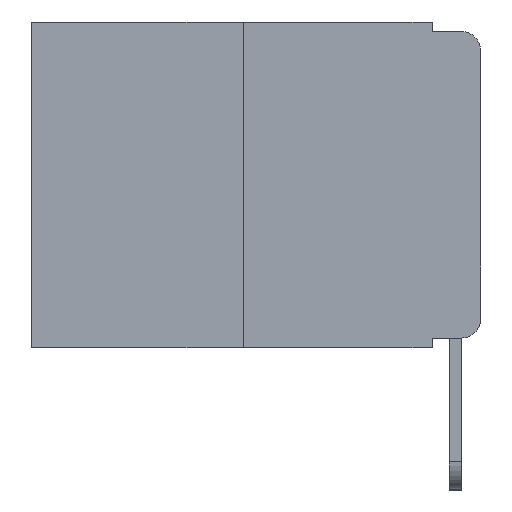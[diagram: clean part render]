
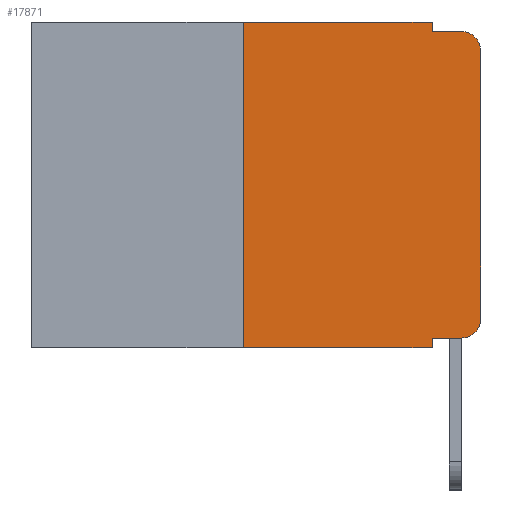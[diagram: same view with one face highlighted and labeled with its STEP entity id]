
A CAD part, left-side view. The second image highlights one B-rep face of the part: STEP entity #17871.
In plain terms, the highlighted planar face has unit normal (-1, 0, 0).
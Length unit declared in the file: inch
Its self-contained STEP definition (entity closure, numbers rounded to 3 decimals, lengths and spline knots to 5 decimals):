
#8 = LINE ( 'NONE', #16566, #3034 ) ;
#457 = CARTESIAN_POINT ( 'NONE',  ( 0., 0.051, -0.01 ) ) ;
#621 = LINE ( 'NONE', #14310, #1189 ) ;
#1189 = VECTOR ( 'NONE', #15718, 39.37008 ) ;
#1249 = CARTESIAN_POINT ( 'NONE',  ( 0., 0., 0. ) ) ;
#1727 = CARTESIAN_POINT ( 'NONE',  ( 0., 0.02, -0.313 ) ) ;
#2177 = VECTOR ( 'NONE', #5731, 39.37008 ) ;
#3034 = VECTOR ( 'NONE', #15217, 39.37008 ) ;
#3135 = EDGE_CURVE ( 'NONE', #12531, #7439, #15941, .T. ) ;
#3433 = DIRECTION ( 'NONE',  ( 0., 0., -1. ) ) ;
#3461 = LINE ( 'NONE', #19270, #11215 ) ;
#3572 = DIRECTION ( 'NONE',  ( -1., 0., 0. ) ) ;
#3809 = VECTOR ( 'NONE', #9124, 39.37008 ) ;
#3925 = AXIS2_PLACEMENT_3D ( 'NONE', #12730, #3572, #14118 ) ;
#3945 = CARTESIAN_POINT ( 'NONE',  ( 0., 0.051, -0.333 ) ) ;
#4028 = EDGE_CURVE ( 'NONE', #7425, #12531, #621, .T. ) ;
#4112 = CARTESIAN_POINT ( 'NONE',  ( 0., 0.473, -0.343 ) ) ;
#4189 = EDGE_CURVE ( 'NONE', #8788, #12583, #12897, .T. ) ;
#4207 = DIRECTION ( 'NONE',  ( 1., 0., 0. ) ) ;
#4212 = EDGE_CURVE ( 'NONE', #7425, #6021, #8064, .T. ) ;
#4279 = EDGE_CURVE ( 'NONE', #8170, #9615, #14399, .T. ) ;
#4402 = EDGE_CURVE ( 'NONE', #8011, #8170, #8, .T. ) ;
#4475 = CARTESIAN_POINT ( 'NONE',  ( 0., 0.051, -0.01 ) ) ;
#4486 = EDGE_CURVE ( 'NONE', #10706, #9615, #5321, .T. ) ;
#4661 = ORIENTED_EDGE ( 'NONE', *, *, #4817, .T. ) ;
#4817 = EDGE_CURVE ( 'NONE', #7439, #10706, #12404, .T. ) ;
#4919 = ORIENTED_EDGE ( 'NONE', *, *, #4486, .T. ) ;
#4971 = ORIENTED_EDGE ( 'NONE', *, *, #4279, .F. ) ;
#4997 = ORIENTED_EDGE ( 'NONE', *, *, #4402, .F. ) ;
#5136 = ORIENTED_EDGE ( 'NONE', *, *, #6971, .F. ) ;
#5210 = ORIENTED_EDGE ( 'NONE', *, *, #4189, .F. ) ;
#5317 = ORIENTED_EDGE ( 'NONE', *, *, #6192, .T. ) ;
#5321 = CIRCLE ( 'NONE', #3925, 0.02 ) ;
#5418 = ORIENTED_EDGE ( 'NONE', *, *, #4212, .F. ) ;
#5472 = ORIENTED_EDGE ( 'NONE', *, *, #4028, .T. ) ;
#5562 = ORIENTED_EDGE ( 'NONE', *, *, #3135, .T. ) ;
#5731 = DIRECTION ( 'NONE',  ( 0., -1., 0. ) ) ;
#5783 = CARTESIAN_POINT ( 'NONE',  ( 0., 0.473, 0. ) ) ;
#6021 = VERTEX_POINT ( 'NONE', #14994 ) ;
#6192 = EDGE_CURVE ( 'NONE', #8788, #6021, #17935, .T. ) ;
#6971 = EDGE_CURVE ( 'NONE', #12583, #8011, #3461, .T. ) ;
#7425 = VERTEX_POINT ( 'NONE', #3945 ) ;
#7439 = VERTEX_POINT ( 'NONE', #14464 ) ;
#7658 = CARTESIAN_POINT ( 'NONE',  ( 0., 0., -0.03 ) ) ;
#8011 = VERTEX_POINT ( 'NONE', #12427 ) ;
#8064 = LINE ( 'NONE', #17441, #3809 ) ;
#8170 = VERTEX_POINT ( 'NONE', #457 ) ;
#8788 = VERTEX_POINT ( 'NONE', #16929 ) ;
#8940 = PLANE ( 'NONE',  #15896 ) ;
#9071 = DIRECTION ( 'NONE',  ( 0., 0., 1. ) ) ;
#9124 = DIRECTION ( 'NONE',  ( 0., 0., -1. ) ) ;
#9615 = VERTEX_POINT ( 'NONE', #10333 ) ;
#10333 = CARTESIAN_POINT ( 'NONE',  ( 0., 0.02, -0.01 ) ) ;
#10401 = FACE_OUTER_BOUND ( 'NONE', #13554, .T. ) ;
#10706 = VERTEX_POINT ( 'NONE', #7658 ) ;
#11215 = VECTOR ( 'NONE', #18028, 39.37008 ) ;
#12404 = LINE ( 'NONE', #1249, #19163 ) ;
#12427 = CARTESIAN_POINT ( 'NONE',  ( 0., 0.051, 0. ) ) ;
#12531 = VERTEX_POINT ( 'NONE', #16753 ) ;
#12583 = VERTEX_POINT ( 'NONE', #12743 ) ;
#12615 = DIRECTION ( 'NONE',  ( -1., 0., 0. ) ) ;
#12730 = CARTESIAN_POINT ( 'NONE',  ( 0., 0.02, -0.03 ) ) ;
#12743 = CARTESIAN_POINT ( 'NONE',  ( 0., 0.25, 0. ) ) ;
#12897 = LINE ( 'NONE', #16127, #19200 ) ;
#13554 = EDGE_LOOP ( 'NONE', ( #4661, #4919, #4971, #4997, #5136, #5210, #5317, #5418, #5472, #5562 ) ) ;
#13976 = VECTOR ( 'NONE', #18924, 39.37008 ) ;
#14118 = DIRECTION ( 'NONE',  ( 0., 0., -1. ) ) ;
#14310 = CARTESIAN_POINT ( 'NONE',  ( 0., 0.051, -0.333 ) ) ;
#14399 = LINE ( 'NONE', #4475, #13976 ) ;
#14464 = CARTESIAN_POINT ( 'NONE',  ( 0., 0., -0.313 ) ) ;
#14687 = DIRECTION ( 'NONE',  ( 0., 0., -1. ) ) ;
#14994 = CARTESIAN_POINT ( 'NONE',  ( 0., 0.051, -0.343 ) ) ;
#15217 = DIRECTION ( 'NONE',  ( 0., 0., -1. ) ) ;
#15718 = DIRECTION ( 'NONE',  ( 0., -1., 0. ) ) ;
#15896 = AXIS2_PLACEMENT_3D ( 'NONE', #5783, #4207, #14687 ) ;
#15941 = CIRCLE ( 'NONE', #18750, 0.02 ) ;
#16127 = CARTESIAN_POINT ( 'NONE',  ( 0., 0.25, 0. ) ) ;
#16566 = CARTESIAN_POINT ( 'NONE',  ( 0., 0.051, 0. ) ) ;
#16753 = CARTESIAN_POINT ( 'NONE',  ( 0., 0.02, -0.333 ) ) ;
#16929 = CARTESIAN_POINT ( 'NONE',  ( 0., 0.25, -0.343 ) ) ;
#17441 = CARTESIAN_POINT ( 'NONE',  ( 0., 0.051, 0. ) ) ;
#17649 = DIRECTION ( 'NONE',  ( 0., 0., 1. ) ) ;
#17871 = ADVANCED_FACE ( 'NONE', ( #10401 ), #8940, .F. ) ;
#17935 = LINE ( 'NONE', #4112, #2177 ) ;
#18028 = DIRECTION ( 'NONE',  ( 0., -1., 0. ) ) ;
#18750 = AXIS2_PLACEMENT_3D ( 'NONE', #1727, #12615, #3433 ) ;
#18924 = DIRECTION ( 'NONE',  ( 0., -1., 0. ) ) ;
#19163 = VECTOR ( 'NONE', #17649, 39.37008 ) ;
#19200 = VECTOR ( 'NONE', #9071, 39.37008 ) ;
#19270 = CARTESIAN_POINT ( 'NONE',  ( 0., 0.473, 0. ) ) ;
